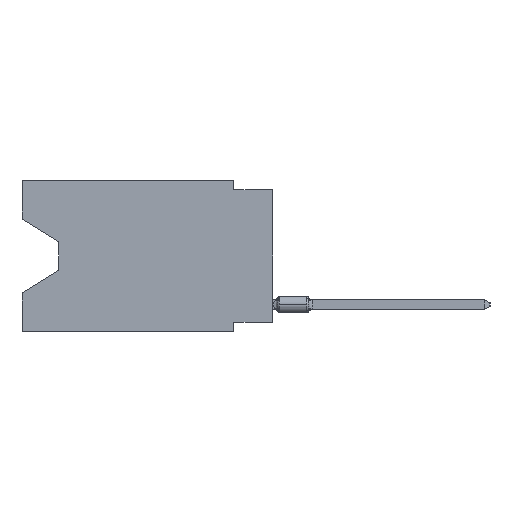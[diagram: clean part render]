
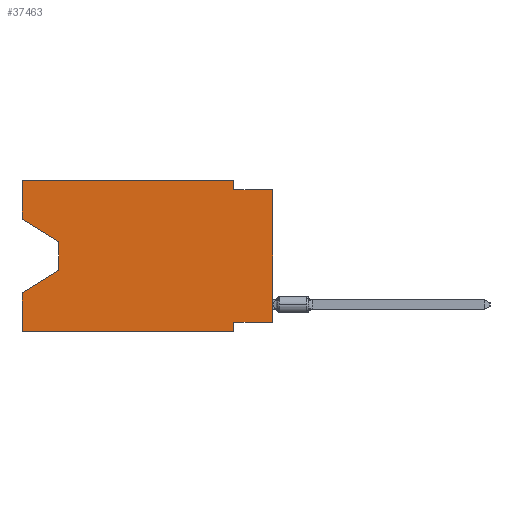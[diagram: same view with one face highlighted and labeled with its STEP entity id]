
A CAD part, left-side view. The second image highlights one B-rep face of the part: STEP entity #37463.
In plain terms, the highlighted planar face has unit normal (-1, 0, 0).
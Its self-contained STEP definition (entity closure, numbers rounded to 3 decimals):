
#419 = CARTESIAN_POINT ( 'NONE',  ( 0., 13.97, -5.893 ) ) ;
#748 = LINE ( 'NONE', #48263, #8088 ) ;
#1165 = VECTOR ( 'NONE', #3544, 1000. ) ;
#1192 = EDGE_CURVE ( 'NONE', #34427, #41525, #748, .T. ) ;
#1258 = VERTEX_POINT ( 'NONE', #19147 ) ;
#3113 = DIRECTION ( 'NONE',  ( 0., -0.855, -0.519 ) ) ;
#3295 = CARTESIAN_POINT ( 'NONE',  ( 0., 2.54, -9.906 ) ) ;
#3544 = DIRECTION ( 'NONE',  ( 0., 0., -1. ) ) ;
#3590 = DIRECTION ( 'NONE',  ( 0., -1., 0. ) ) ;
#4779 = CARTESIAN_POINT ( 'NONE',  ( 0., 2.54, 0. ) ) ;
#5463 = DIRECTION ( 'NONE',  ( 1., 0., 0. ) ) ;
#6063 = VERTEX_POINT ( 'NONE', #27242 ) ;
#6078 = ORIENTED_EDGE ( 'NONE', *, *, #35538, .F. ) ;
#6537 = ORIENTED_EDGE ( 'NONE', *, *, #12724, .F. ) ;
#6847 = VECTOR ( 'NONE', #11171, 1000. ) ;
#8088 = VECTOR ( 'NONE', #41652, 1000. ) ;
#8363 = VERTEX_POINT ( 'NONE', #15928 ) ;
#8609 = VECTOR ( 'NONE', #23945, 1000. ) ;
#8801 = VECTOR ( 'NONE', #37104, 1000. ) ;
#9155 = FACE_OUTER_BOUND ( 'NONE', #16374, .T. ) ;
#9181 = LINE ( 'NONE', #35369, #41965 ) ;
#9844 = EDGE_CURVE ( 'NONE', #1258, #31211, #18086, .T. ) ;
#10681 = VERTEX_POINT ( 'NONE', #19838 ) ;
#11171 = DIRECTION ( 'NONE',  ( 0., 0., -1. ) ) ;
#11392 = EDGE_CURVE ( 'NONE', #12790, #41525, #37355, .T. ) ;
#11547 = AXIS2_PLACEMENT_3D ( 'NONE', #16769, #5463, #48299 ) ;
#11683 = LINE ( 'NONE', #29798, #35758 ) ;
#12463 = CARTESIAN_POINT ( 'NONE',  ( 0., 0., -9.271 ) ) ;
#12724 = EDGE_CURVE ( 'NONE', #1258, #38580, #41087, .T. ) ;
#12790 = VERTEX_POINT ( 'NONE', #419 ) ;
#13822 = CARTESIAN_POINT ( 'NONE',  ( 0., 16.383, 0. ) ) ;
#14501 = EDGE_CURVE ( 'NONE', #6063, #31759, #42007, .T. ) ;
#14599 = EDGE_CURVE ( 'NONE', #10681, #31759, #9181, .T. ) ;
#15568 = CARTESIAN_POINT ( 'NONE',  ( 0., 16.383, -9.906 ) ) ;
#15928 = CARTESIAN_POINT ( 'NONE',  ( 0., 2.54, -9.906 ) ) ;
#16084 = CARTESIAN_POINT ( 'NONE',  ( 0., 0., 0. ) ) ;
#16374 = EDGE_LOOP ( 'NONE', ( #29524, #19827, #41193, #22224, #30918, #30835, #32739, #44605, #30019, #41401, #6078, #6537 ) ) ;
#16769 = CARTESIAN_POINT ( 'NONE',  ( 0., 16.383, 0. ) ) ;
#17098 = VERTEX_POINT ( 'NONE', #24649 ) ;
#17318 = EDGE_CURVE ( 'NONE', #47049, #10681, #22441, .T. ) ;
#18086 = LINE ( 'NONE', #37407, #26660 ) ;
#19147 = CARTESIAN_POINT ( 'NONE',  ( 0., 16.383, -2.546 ) ) ;
#19827 = ORIENTED_EDGE ( 'NONE', *, *, #26787, .T. ) ;
#19838 = CARTESIAN_POINT ( 'NONE',  ( 0., 2.54, -0.635 ) ) ;
#22224 = ORIENTED_EDGE ( 'NONE', *, *, #1192, .F. ) ;
#22441 = LINE ( 'NONE', #4779, #6847 ) ;
#22648 = LINE ( 'NONE', #15568, #28416 ) ;
#23708 = LINE ( 'NONE', #12463, #8609 ) ;
#23945 = DIRECTION ( 'NONE',  ( 0., 1., 0. ) ) ;
#24094 = PLANE ( 'NONE',  #11547 ) ;
#24592 = EDGE_CURVE ( 'NONE', #17098, #8363, #26066, .T. ) ;
#24649 = CARTESIAN_POINT ( 'NONE',  ( 0., 2.54, -9.271 ) ) ;
#25356 = CARTESIAN_POINT ( 'NONE',  ( 0., 16.383, -7.36 ) ) ;
#25990 = CARTESIAN_POINT ( 'NONE',  ( 0., 2.54, 0. ) ) ;
#26066 = LINE ( 'NONE', #3295, #1165 ) ;
#26335 = VECTOR ( 'NONE', #44342, 1000. ) ;
#26660 = VECTOR ( 'NONE', #3113, 1000. ) ;
#26787 = EDGE_CURVE ( 'NONE', #31211, #12790, #29377, .T. ) ;
#27242 = CARTESIAN_POINT ( 'NONE',  ( 0., 0., -9.271 ) ) ;
#28364 = CARTESIAN_POINT ( 'NONE',  ( 0., 13.97, -4.013 ) ) ;
#28416 = VECTOR ( 'NONE', #30452, 1000. ) ;
#29377 = LINE ( 'NONE', #41398, #26335 ) ;
#29524 = ORIENTED_EDGE ( 'NONE', *, *, #9844, .T. ) ;
#29798 = CARTESIAN_POINT ( 'NONE',  ( 0., 16.383, 0. ) ) ;
#30019 = ORIENTED_EDGE ( 'NONE', *, *, #14599, .F. ) ;
#30452 = DIRECTION ( 'NONE',  ( 0., -1., 0. ) ) ;
#30835 = ORIENTED_EDGE ( 'NONE', *, *, #24592, .F. ) ;
#30918 = ORIENTED_EDGE ( 'NONE', *, *, #32356, .T. ) ;
#31211 = VERTEX_POINT ( 'NONE', #28364 ) ;
#31547 = EDGE_CURVE ( 'NONE', #6063, #17098, #23708, .T. ) ;
#31759 = VERTEX_POINT ( 'NONE', #40315 ) ;
#32356 = EDGE_CURVE ( 'NONE', #34427, #8363, #22648, .T. ) ;
#32739 = ORIENTED_EDGE ( 'NONE', *, *, #31547, .F. ) ;
#34427 = VERTEX_POINT ( 'NONE', #46973 ) ;
#35369 = CARTESIAN_POINT ( 'NONE',  ( 0., 0., -0.635 ) ) ;
#35538 = EDGE_CURVE ( 'NONE', #38580, #47049, #11683, .T. ) ;
#35758 = VECTOR ( 'NONE', #3590, 1000. ) ;
#37104 = DIRECTION ( 'NONE',  ( 0., 0.855, -0.519 ) ) ;
#37355 = LINE ( 'NONE', #44710, #8801 ) ;
#37407 = CARTESIAN_POINT ( 'NONE',  ( 0., 16.383, -2.546 ) ) ;
#37463 = ADVANCED_FACE ( 'NONE', ( #9155 ), #24094, .F. ) ;
#38580 = VERTEX_POINT ( 'NONE', #13822 ) ;
#40315 = CARTESIAN_POINT ( 'NONE',  ( 0., 0., -0.635 ) ) ;
#40841 = CARTESIAN_POINT ( 'NONE',  ( 0., 16.383, 0. ) ) ;
#41087 = LINE ( 'NONE', #40841, #44039 ) ;
#41193 = ORIENTED_EDGE ( 'NONE', *, *, #11392, .T. ) ;
#41398 = CARTESIAN_POINT ( 'NONE',  ( 0., 13.97, -4.013 ) ) ;
#41401 = ORIENTED_EDGE ( 'NONE', *, *, #17318, .F. ) ;
#41525 = VERTEX_POINT ( 'NONE', #25356 ) ;
#41652 = DIRECTION ( 'NONE',  ( 0., 0., 1. ) ) ;
#41965 = VECTOR ( 'NONE', #46166, 1000. ) ;
#42007 = LINE ( 'NONE', #16084, #42740 ) ;
#42740 = VECTOR ( 'NONE', #45688, 1000. ) ;
#44039 = VECTOR ( 'NONE', #47940, 1000. ) ;
#44342 = DIRECTION ( 'NONE',  ( 0., 0., -1. ) ) ;
#44605 = ORIENTED_EDGE ( 'NONE', *, *, #14501, .T. ) ;
#44710 = CARTESIAN_POINT ( 'NONE',  ( 0., 13.97, -5.893 ) ) ;
#45688 = DIRECTION ( 'NONE',  ( 0., 0., 1. ) ) ;
#46166 = DIRECTION ( 'NONE',  ( 0., -1., 0. ) ) ;
#46973 = CARTESIAN_POINT ( 'NONE',  ( 0., 16.383, -9.906 ) ) ;
#47049 = VERTEX_POINT ( 'NONE', #25990 ) ;
#47940 = DIRECTION ( 'NONE',  ( 0., 0., 1. ) ) ;
#48263 = CARTESIAN_POINT ( 'NONE',  ( 0., 16.383, 0. ) ) ;
#48299 = DIRECTION ( 'NONE',  ( 0., 0., -1. ) ) ;
